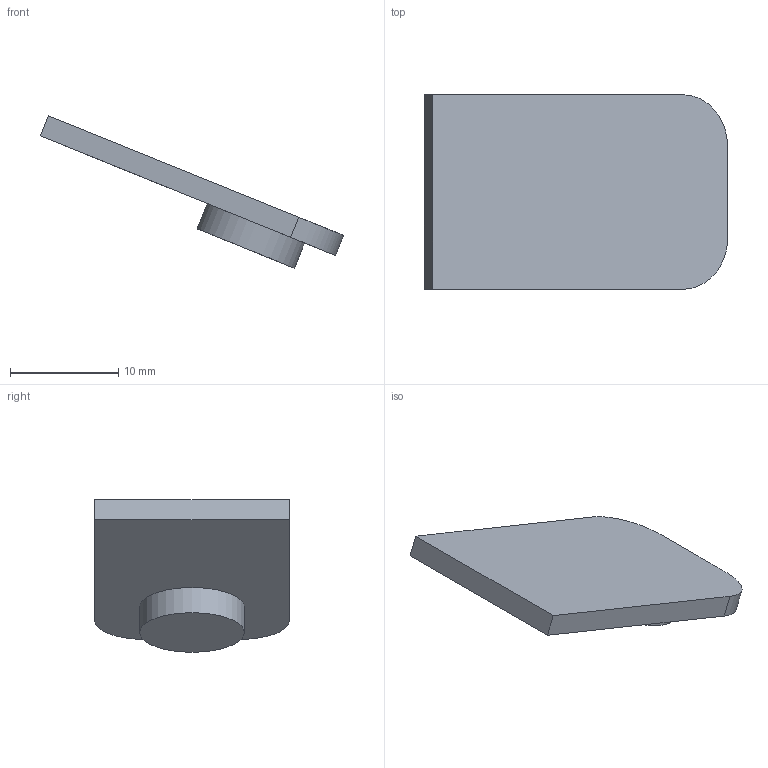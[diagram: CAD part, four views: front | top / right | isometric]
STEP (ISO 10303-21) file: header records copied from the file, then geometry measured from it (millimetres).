
FILE_DESCRIPTION(/* description */ (''),/* implementation_level */ '2;1');
FILE_NAME(/* name */ 'Locking Tab.step',/* time_stamp */ '2022-05-12T10:52:50-06:00',/* author */ (''),/* organization */ (''),/* preprocessor_version */ 'ST-DEVELOPER v18.1',/* originating_system */ 'Autodesk Translation Framework v10.10.0.1391',/* authorisation */ '');
FILE_SCHEMA (('AUTOMOTIVE_DESIGN { 1 0 10303 214 3 1 1 }'));
Length unit declared in the file: millimetre
Products named in the file (1): locking tab
Bounding box: 28.02 x 17.98 x 14.09 mm (x, y, z)
Volume: 1226.3 mm3; surface area: 1298.6 mm2
Topology: 1 solids, 1 shells, 10 faces, 21 edges, 14 vertices
Faces by surface type: plane 7, bspline 2, cylinder 1
Full cylindrical faces by diameter (mm): 9.7 x1
Entity records: 396 total; most frequent: CARTESIAN_POINT 156, ORIENTED_EDGE 42, DIRECTION 37, EDGE_CURVE 21, LINE 15, VECTOR 15, VERTEX_POINT 14, EDGE_LOOP 11
